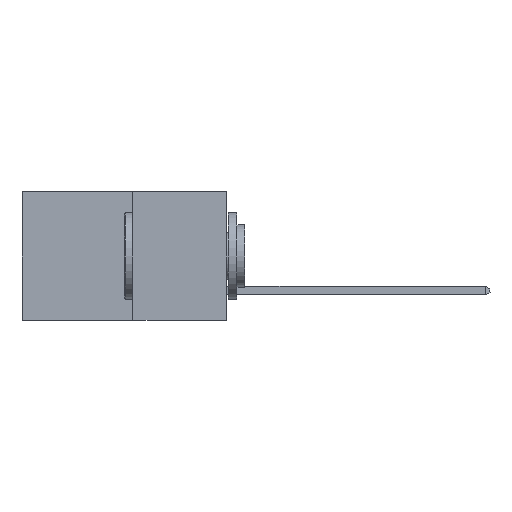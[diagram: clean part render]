
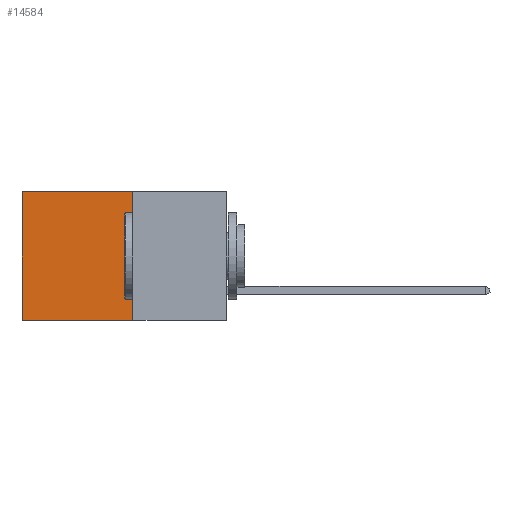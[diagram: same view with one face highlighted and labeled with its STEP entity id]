
A CAD part, left-side view. The second image highlights one B-rep face of the part: STEP entity #14584.
In plain terms, the highlighted planar face has unit normal (-1, 0, 0).
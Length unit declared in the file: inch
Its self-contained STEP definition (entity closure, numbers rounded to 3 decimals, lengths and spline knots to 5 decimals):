
#309 = CARTESIAN_POINT ( 'NONE',  ( 0.277, 0.27, -0.37 ) ) ;
#1278 = LINE ( 'NONE', #10174, #14705 ) ;
#1789 = EDGE_CURVE ( 'NONE', #10870, #13078, #1278, .T. ) ;
#2563 = VERTEX_POINT ( 'NONE', #14621 ) ;
#2856 = CARTESIAN_POINT ( 'NONE',  ( 0.277, 0.27, -0.37 ) ) ;
#3081 = DIRECTION ( 'NONE',  ( 0., 0., -1. ) ) ;
#3085 = LINE ( 'NONE', #8697, #16392 ) ;
#3112 = FACE_OUTER_BOUND ( 'NONE', #12687, .T. ) ;
#3442 = CARTESIAN_POINT ( 'NONE',  ( 0.277, 0.59, -0.37 ) ) ;
#4466 = AXIS2_PLACEMENT_3D ( 'NONE', #309, #10911, #3081 ) ;
#5298 = CARTESIAN_POINT ( 'NONE',  ( 0.277, 0.59, -0.37 ) ) ;
#5462 = EDGE_CURVE ( 'NONE', #15488, #13078, #15539, .T. ) ;
#5895 = VECTOR ( 'NONE', #10699, 39.37008 ) ;
#6059 = ORIENTED_EDGE ( 'NONE', *, *, #5462, .T. ) ;
#7443 = ORIENTED_EDGE ( 'NONE', *, *, #11550, .F. ) ;
#8697 = CARTESIAN_POINT ( 'NONE',  ( 0.277, 0.27, 0. ) ) ;
#9799 = LINE ( 'NONE', #2856, #5895 ) ;
#10001 = DIRECTION ( 'NONE',  ( 0., 1., 0. ) ) ;
#10049 = DIRECTION ( 'NONE',  ( 0., 0., -1. ) ) ;
#10174 = CARTESIAN_POINT ( 'NONE',  ( 0.277, 0.27, -0.37 ) ) ;
#10699 = DIRECTION ( 'NONE',  ( 0., 0., -1. ) ) ;
#10870 = VERTEX_POINT ( 'NONE', #14306 ) ;
#10911 = DIRECTION ( 'NONE',  ( 1., 0., 0. ) ) ;
#11519 = DIRECTION ( 'NONE',  ( 0., 1., 0. ) ) ;
#11550 = EDGE_CURVE ( 'NONE', #2563, #10870, #9799, .T. ) ;
#12221 = VECTOR ( 'NONE', #10049, 39.37008 ) ;
#12687 = EDGE_LOOP ( 'NONE', ( #6059, #14661, #7443, #16533 ) ) ;
#13078 = VERTEX_POINT ( 'NONE', #5298 ) ;
#14306 = CARTESIAN_POINT ( 'NONE',  ( 0.277, 0.27, -0.37 ) ) ;
#14584 = ADVANCED_FACE ( 'NONE', ( #3112 ), #15933, .F. ) ;
#14621 = CARTESIAN_POINT ( 'NONE',  ( 0.277, 0.27, 0. ) ) ;
#14661 = ORIENTED_EDGE ( 'NONE', *, *, #1789, .F. ) ;
#14705 = VECTOR ( 'NONE', #11519, 39.37008 ) ;
#15488 = VERTEX_POINT ( 'NONE', #16298 ) ;
#15496 = EDGE_CURVE ( 'NONE', #2563, #15488, #3085, .T. ) ;
#15539 = LINE ( 'NONE', #3442, #12221 ) ;
#15933 = PLANE ( 'NONE',  #4466 ) ;
#16298 = CARTESIAN_POINT ( 'NONE',  ( 0.277, 0.59, 0. ) ) ;
#16392 = VECTOR ( 'NONE', #10001, 39.37008 ) ;
#16533 = ORIENTED_EDGE ( 'NONE', *, *, #15496, .T. ) ;
